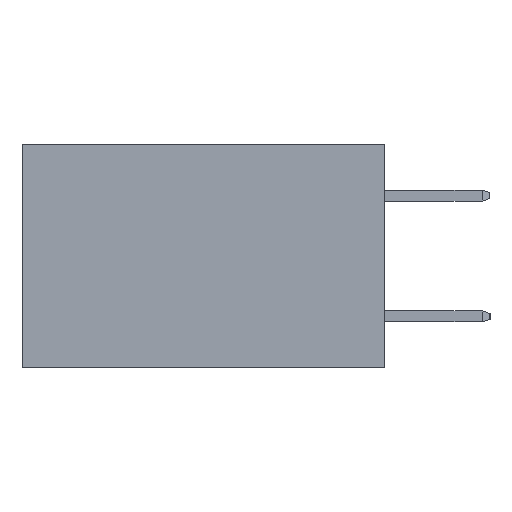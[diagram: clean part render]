
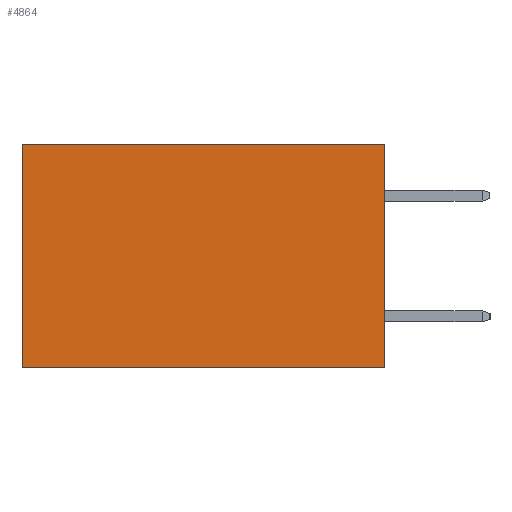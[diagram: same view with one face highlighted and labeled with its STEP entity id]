
A CAD part, left-side view. The second image highlights one B-rep face of the part: STEP entity #4864.
In plain terms, the highlighted planar face has unit normal (-1, 0, 0).
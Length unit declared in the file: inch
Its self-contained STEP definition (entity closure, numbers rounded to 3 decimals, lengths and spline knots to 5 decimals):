
#1437 = VERTEX_POINT ( 'NONE', #6399 ) ;
#1513 = DIRECTION ( 'NONE',  ( 0., 0., -1. ) ) ;
#1610 = DIRECTION ( 'NONE',  ( 1., 0., 0. ) ) ;
#1869 = PLANE ( 'NONE',  #8659 ) ;
#1896 = ORIENTED_EDGE ( 'NONE', *, *, #8986, .F. ) ;
#2079 = LINE ( 'NONE', #9472, #12286 ) ;
#2409 = EDGE_CURVE ( 'NONE', #5661, #10498, #10886, .T. ) ;
#3343 = DIRECTION ( 'NONE',  ( 0., 1., 0. ) ) ;
#3401 = ORIENTED_EDGE ( 'NONE', *, *, #9047, .T. ) ;
#3919 = CARTESIAN_POINT ( 'NONE',  ( 0.2615, 0., -0.37 ) ) ;
#4864 = ADVANCED_FACE ( 'NONE', ( #5653 ), #1869, .F. ) ;
#4887 = LINE ( 'NONE', #10007, #11491 ) ;
#5264 = EDGE_LOOP ( 'NONE', ( #8672, #12817, #1896, #3401 ) ) ;
#5465 = DIRECTION ( 'NONE',  ( 0., 0., -1. ) ) ;
#5653 = FACE_OUTER_BOUND ( 'NONE', #5264, .T. ) ;
#5661 = VERTEX_POINT ( 'NONE', #10127 ) ;
#5752 = CARTESIAN_POINT ( 'NONE',  ( 0.2615, 0.6, -0.37 ) ) ;
#6399 = CARTESIAN_POINT ( 'NONE',  ( 0.2615, 0., 0. ) ) ;
#6508 = VECTOR ( 'NONE', #12594, 39.37008 ) ;
#7199 = DIRECTION ( 'NONE',  ( 0., 1., 0. ) ) ;
#7299 = CARTESIAN_POINT ( 'NONE',  ( 0.2615, 0., -0.37 ) ) ;
#8023 = VERTEX_POINT ( 'NONE', #7299 ) ;
#8659 = AXIS2_PLACEMENT_3D ( 'NONE', #3919, #1610, #1513 ) ;
#8672 = ORIENTED_EDGE ( 'NONE', *, *, #2409, .T. ) ;
#8986 = EDGE_CURVE ( 'NONE', #1437, #8023, #10425, .T. ) ;
#9047 = EDGE_CURVE ( 'NONE', #1437, #5661, #2079, .T. ) ;
#9472 = CARTESIAN_POINT ( 'NONE',  ( 0.2615, 0., 0. ) ) ;
#10007 = CARTESIAN_POINT ( 'NONE',  ( 0.2615, 0., -0.37 ) ) ;
#10127 = CARTESIAN_POINT ( 'NONE',  ( 0.2615, 0.6, 0. ) ) ;
#10425 = LINE ( 'NONE', #12487, #6508 ) ;
#10498 = VERTEX_POINT ( 'NONE', #11557 ) ;
#10886 = LINE ( 'NONE', #5752, #13945 ) ;
#11491 = VECTOR ( 'NONE', #3343, 39.37008 ) ;
#11557 = CARTESIAN_POINT ( 'NONE',  ( 0.2615, 0.6, -0.37 ) ) ;
#12286 = VECTOR ( 'NONE', #7199, 39.37008 ) ;
#12487 = CARTESIAN_POINT ( 'NONE',  ( 0.2615, 0., -0.37 ) ) ;
#12594 = DIRECTION ( 'NONE',  ( 0., 0., -1. ) ) ;
#12817 = ORIENTED_EDGE ( 'NONE', *, *, #16599, .F. ) ;
#13945 = VECTOR ( 'NONE', #5465, 39.37008 ) ;
#16599 = EDGE_CURVE ( 'NONE', #8023, #10498, #4887, .T. ) ;
